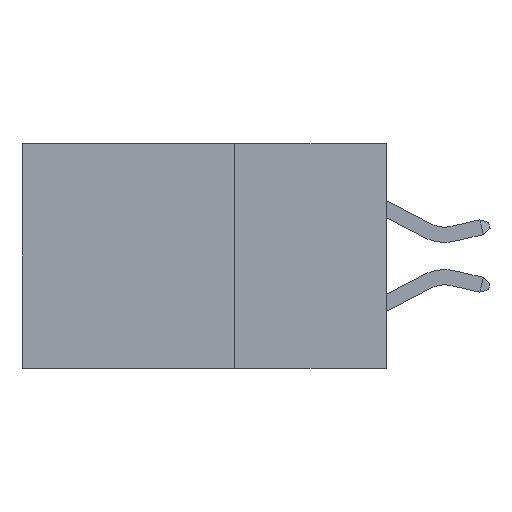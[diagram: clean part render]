
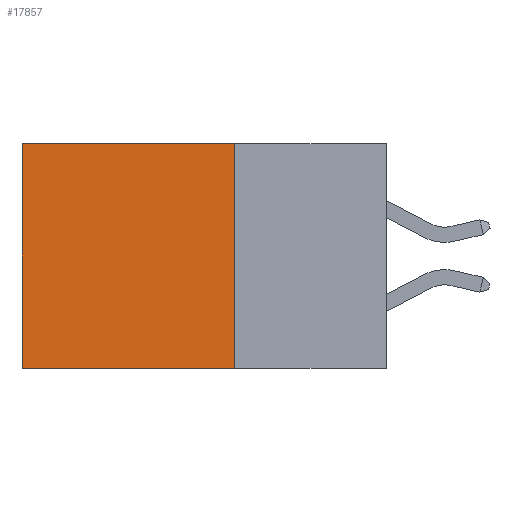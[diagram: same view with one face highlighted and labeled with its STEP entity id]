
A CAD part, left-side view. The second image highlights one B-rep face of the part: STEP entity #17857.
In plain terms, the highlighted planar face has unit normal (-1, 0, 0).
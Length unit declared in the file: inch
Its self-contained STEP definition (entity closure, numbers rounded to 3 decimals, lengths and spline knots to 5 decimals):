
#862 = CARTESIAN_POINT ( 'NONE',  ( 0.298, 0.25, 0. ) ) ;
#973 = VERTEX_POINT ( 'NONE', #24949 ) ;
#1667 = VERTEX_POINT ( 'NONE', #12736 ) ;
#2770 = DIRECTION ( 'NONE',  ( 0., 1., 0. ) ) ;
#3983 = DIRECTION ( 'NONE',  ( 0., 0., -1. ) ) ;
#5186 = ORIENTED_EDGE ( 'NONE', *, *, #15261, .F. ) ;
#5284 = ORIENTED_EDGE ( 'NONE', *, *, #16896, .F. ) ;
#6011 = CARTESIAN_POINT ( 'NONE',  ( 0.298, 0.25, -0.37 ) ) ;
#6041 = LINE ( 'NONE', #14907, #24728 ) ;
#6512 = PLANE ( 'NONE',  #16385 ) ;
#7505 = LINE ( 'NONE', #13682, #18935 ) ;
#8029 = VERTEX_POINT ( 'NONE', #6011 ) ;
#8817 = LINE ( 'NONE', #21162, #14544 ) ;
#8954 = VECTOR ( 'NONE', #30110, 39.37008 ) ;
#8974 = FACE_OUTER_BOUND ( 'NONE', #12238, .T. ) ;
#9005 = DIRECTION ( 'NONE',  ( 0., 0., -1. ) ) ;
#11431 = DIRECTION ( 'NONE',  ( 0., 0., -1. ) ) ;
#12238 = EDGE_LOOP ( 'NONE', ( #21168, #5284, #5186, #20630 ) ) ;
#12343 = EDGE_CURVE ( 'NONE', #973, #21760, #21927, .T. ) ;
#12736 = CARTESIAN_POINT ( 'NONE',  ( 0.298, 0.6, -0.37 ) ) ;
#13450 = CARTESIAN_POINT ( 'NONE',  ( 0.298, 0.6, 0. ) ) ;
#13682 = CARTESIAN_POINT ( 'NONE',  ( 0.298, 0.6, 0. ) ) ;
#14544 = VECTOR ( 'NONE', #9005, 39.37008 ) ;
#14907 = CARTESIAN_POINT ( 'NONE',  ( 0.298, 0.25, -0.37 ) ) ;
#15261 = EDGE_CURVE ( 'NONE', #973, #8029, #8817, .T. ) ;
#16385 = AXIS2_PLACEMENT_3D ( 'NONE', #23584, #26051, #11431 ) ;
#16896 = EDGE_CURVE ( 'NONE', #8029, #1667, #6041, .T. ) ;
#17857 = ADVANCED_FACE ( 'NONE', ( #8974 ), #6512, .F. ) ;
#18935 = VECTOR ( 'NONE', #3983, 39.37008 ) ;
#20630 = ORIENTED_EDGE ( 'NONE', *, *, #12343, .T. ) ;
#21162 = CARTESIAN_POINT ( 'NONE',  ( 0.298, 0.25, 0. ) ) ;
#21168 = ORIENTED_EDGE ( 'NONE', *, *, #24889, .T. ) ;
#21760 = VERTEX_POINT ( 'NONE', #13450 ) ;
#21927 = LINE ( 'NONE', #862, #8954 ) ;
#23584 = CARTESIAN_POINT ( 'NONE',  ( 0.298, 0.25, 0. ) ) ;
#24728 = VECTOR ( 'NONE', #2770, 39.37008 ) ;
#24889 = EDGE_CURVE ( 'NONE', #21760, #1667, #7505, .T. ) ;
#24949 = CARTESIAN_POINT ( 'NONE',  ( 0.298, 0.25, 0. ) ) ;
#26051 = DIRECTION ( 'NONE',  ( 1., 0., 0. ) ) ;
#30110 = DIRECTION ( 'NONE',  ( 0., 1., 0. ) ) ;
